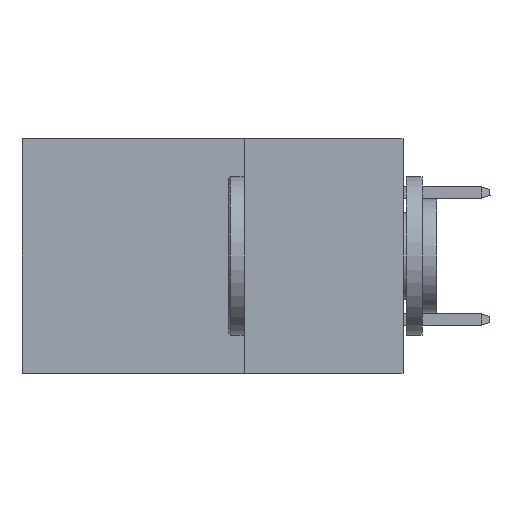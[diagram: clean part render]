
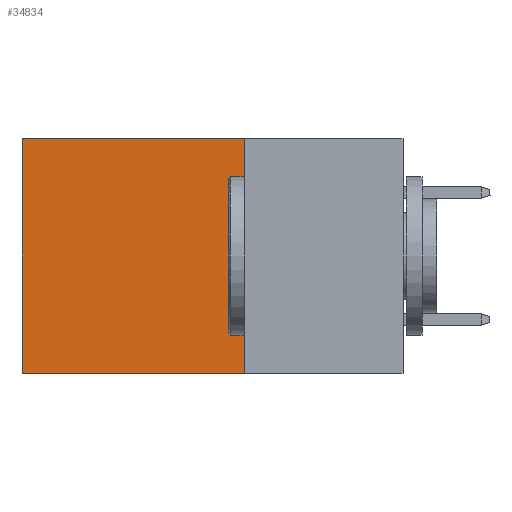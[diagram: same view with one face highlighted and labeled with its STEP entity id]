
A CAD part, left-side view. The second image highlights one B-rep face of the part: STEP entity #34834.
In plain terms, the highlighted planar face has unit normal (-1, 0, 0).
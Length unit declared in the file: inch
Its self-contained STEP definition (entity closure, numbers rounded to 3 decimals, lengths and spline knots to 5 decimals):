
#783 = DIRECTION ( 'NONE',  ( 0., 0., -1. ) ) ;
#1143 = LINE ( 'NONE', #30899, #27260 ) ;
#1196 = CARTESIAN_POINT ( 'NONE',  ( 0.2875, 0.25, 0. ) ) ;
#2456 = VECTOR ( 'NONE', #783, 39.37008 ) ;
#4632 = CARTESIAN_POINT ( 'NONE',  ( 0.2875, 0.25, 0. ) ) ;
#5237 = EDGE_CURVE ( 'NONE', #9963, #33868, #1143, .T. ) ;
#6112 = CARTESIAN_POINT ( 'NONE',  ( 0.2875, 0.6, -0.37 ) ) ;
#6156 = PLANE ( 'NONE',  #23526 ) ;
#6513 = DIRECTION ( 'NONE',  ( 1., 0., 0. ) ) ;
#6830 = VECTOR ( 'NONE', #20760, 39.37008 ) ;
#6892 = CARTESIAN_POINT ( 'NONE',  ( 0.2875, 0.6, 0. ) ) ;
#8009 = ORIENTED_EDGE ( 'NONE', *, *, #28463, .T. ) ;
#8207 = ORIENTED_EDGE ( 'NONE', *, *, #10828, .F. ) ;
#9818 = VECTOR ( 'NONE', #18703, 39.37008 ) ;
#9963 = VERTEX_POINT ( 'NONE', #27466 ) ;
#10828 = EDGE_CURVE ( 'NONE', #19192, #9963, #14238, .T. ) ;
#14238 = LINE ( 'NONE', #25080, #2456 ) ;
#14310 = DIRECTION ( 'NONE',  ( 0., 0., -1. ) ) ;
#16823 = VERTEX_POINT ( 'NONE', #6892 ) ;
#18703 = DIRECTION ( 'NONE',  ( 0., 0., -1. ) ) ;
#19192 = VERTEX_POINT ( 'NONE', #30368 ) ;
#20760 = DIRECTION ( 'NONE',  ( 0., 1., 0. ) ) ;
#21373 = CARTESIAN_POINT ( 'NONE',  ( 0.2875, 0.6, 0. ) ) ;
#22781 = DIRECTION ( 'NONE',  ( 0., 1., 0. ) ) ;
#23526 = AXIS2_PLACEMENT_3D ( 'NONE', #1196, #6513, #14310 ) ;
#24906 = ORIENTED_EDGE ( 'NONE', *, *, #5237, .F. ) ;
#25080 = CARTESIAN_POINT ( 'NONE',  ( 0.2875, 0.25, 0. ) ) ;
#26882 = LINE ( 'NONE', #21373, #9818 ) ;
#27260 = VECTOR ( 'NONE', #22781, 39.37008 ) ;
#27466 = CARTESIAN_POINT ( 'NONE',  ( 0.2875, 0.25, -0.37 ) ) ;
#28463 = EDGE_CURVE ( 'NONE', #19192, #16823, #28569, .T. ) ;
#28569 = LINE ( 'NONE', #4632, #6830 ) ;
#30368 = CARTESIAN_POINT ( 'NONE',  ( 0.2875, 0.25, 0. ) ) ;
#30444 = FACE_OUTER_BOUND ( 'NONE', #33455, .T. ) ;
#30899 = CARTESIAN_POINT ( 'NONE',  ( 0.2875, 0.25, -0.37 ) ) ;
#30986 = EDGE_CURVE ( 'NONE', #16823, #33868, #26882, .T. ) ;
#31499 = ORIENTED_EDGE ( 'NONE', *, *, #30986, .T. ) ;
#33455 = EDGE_LOOP ( 'NONE', ( #31499, #24906, #8207, #8009 ) ) ;
#33868 = VERTEX_POINT ( 'NONE', #6112 ) ;
#34834 = ADVANCED_FACE ( 'NONE', ( #30444 ), #6156, .F. ) ;
